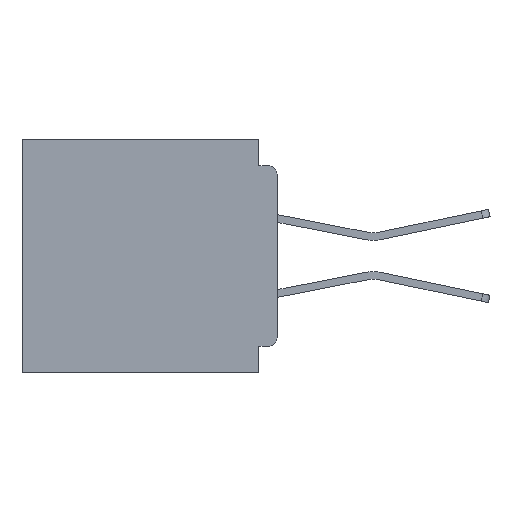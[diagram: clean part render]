
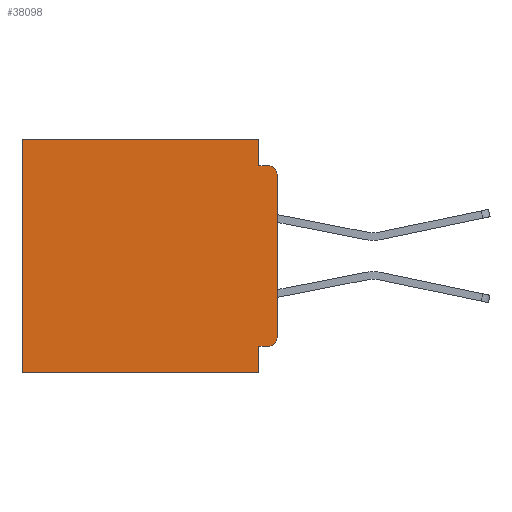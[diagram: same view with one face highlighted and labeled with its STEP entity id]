
A CAD part, left-side view. The second image highlights one B-rep face of the part: STEP entity #38098.
In plain terms, the highlighted planar face has unit normal (-1, 0, 0).
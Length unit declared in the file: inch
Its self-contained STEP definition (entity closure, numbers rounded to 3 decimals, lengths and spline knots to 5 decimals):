
#147 = FACE_OUTER_BOUND ( 'NONE', #43407, .T. ) ;
#606 = EDGE_CURVE ( 'NONE', #39332, #37207, #25156, .T. ) ;
#1272 = CARTESIAN_POINT ( 'NONE',  ( 0.3, 0.437, -0.4 ) ) ;
#1820 = EDGE_CURVE ( 'NONE', #10817, #36808, #22359, .T. ) ;
#2130 = DIRECTION ( 'NONE',  ( 0., 0., -1. ) ) ;
#2560 = ORIENTED_EDGE ( 'NONE', *, *, #606, .F. ) ;
#2570 = DIRECTION ( 'NONE',  ( 0., 0., -1. ) ) ;
#2652 = CIRCLE ( 'NONE', #17089, 0.015 ) ;
#2797 = DIRECTION ( 'NONE',  ( -1., 0., 0. ) ) ;
#3921 = ORIENTED_EDGE ( 'NONE', *, *, #14680, .F. ) ;
#4064 = ORIENTED_EDGE ( 'NONE', *, *, #9618, .T. ) ;
#5972 = DIRECTION ( 'NONE',  ( 0., 0., -1. ) ) ;
#6130 = VERTEX_POINT ( 'NONE', #18935 ) ;
#6526 = DIRECTION ( 'NONE',  ( 0., -1., 0. ) ) ;
#8549 = CARTESIAN_POINT ( 'NONE',  ( 0.3, 0., -0.4 ) ) ;
#8868 = VERTEX_POINT ( 'NONE', #12623 ) ;
#8914 = DIRECTION ( 'NONE',  ( 0., 0., -1. ) ) ;
#9393 = CARTESIAN_POINT ( 'NONE',  ( 0.3, 0.437, 0. ) ) ;
#9618 = EDGE_CURVE ( 'NONE', #10817, #8868, #2652, .T. ) ;
#10704 = VERTEX_POINT ( 'NONE', #26152 ) ;
#10817 = VERTEX_POINT ( 'NONE', #30225 ) ;
#11202 = VECTOR ( 'NONE', #26905, 39.37008 ) ;
#11681 = ORIENTED_EDGE ( 'NONE', *, *, #40359, .T. ) ;
#11682 = CARTESIAN_POINT ( 'NONE',  ( 0.3, 0.031, 0. ) ) ;
#12623 = CARTESIAN_POINT ( 'NONE',  ( 0.3, 0.015, -0.045 ) ) ;
#12744 = CARTESIAN_POINT ( 'NONE',  ( 0.3, 0., -0.4 ) ) ;
#12947 = CARTESIAN_POINT ( 'NONE',  ( 0.3, 0., 0. ) ) ;
#14680 = EDGE_CURVE ( 'NONE', #10704, #8868, #37393, .T. ) ;
#14986 = CARTESIAN_POINT ( 'NONE',  ( 0.3, 0.015, -0.34 ) ) ;
#15662 = EDGE_CURVE ( 'NONE', #21850, #10704, #32672, .T. ) ;
#16188 = CARTESIAN_POINT ( 'NONE',  ( 0.3, 0., -0.34 ) ) ;
#16303 = EDGE_CURVE ( 'NONE', #28092, #37207, #42016, .T. ) ;
#16659 = CARTESIAN_POINT ( 'NONE',  ( 0.3, 0.015, -0.355 ) ) ;
#17089 = AXIS2_PLACEMENT_3D ( 'NONE', #23402, #2797, #26845 ) ;
#17104 = VECTOR ( 'NONE', #6526, 39.37008 ) ;
#18450 = DIRECTION ( 'NONE',  ( 0., 0., -1. ) ) ;
#18935 = CARTESIAN_POINT ( 'NONE',  ( 0.3, 0.031, -0.355 ) ) ;
#19880 = VECTOR ( 'NONE', #36865, 39.37008 ) ;
#19909 = ORIENTED_EDGE ( 'NONE', *, *, #16303, .T. ) ;
#20310 = ORIENTED_EDGE ( 'NONE', *, *, #31011, .F. ) ;
#20761 = EDGE_CURVE ( 'NONE', #22041, #6130, #40576, .T. ) ;
#21850 = VERTEX_POINT ( 'NONE', #11682 ) ;
#22041 = VERTEX_POINT ( 'NONE', #16659 ) ;
#22345 = AXIS2_PLACEMENT_3D ( 'NONE', #14986, #38849, #18450 ) ;
#22359 = LINE ( 'NONE', #8549, #39309 ) ;
#22514 = VECTOR ( 'NONE', #8914, 39.37008 ) ;
#23038 = PLANE ( 'NONE',  #38952 ) ;
#23187 = DIRECTION ( 'NONE',  ( 1., 0., 0. ) ) ;
#23402 = CARTESIAN_POINT ( 'NONE',  ( 0.3, 0.015, -0.06 ) ) ;
#23464 = CARTESIAN_POINT ( 'NONE',  ( 0.3, 0., -0.355 ) ) ;
#24066 = CIRCLE ( 'NONE', #22345, 0.015 ) ;
#25050 = ORIENTED_EDGE ( 'NONE', *, *, #42413, .T. ) ;
#25156 = LINE ( 'NONE', #28033, #33139 ) ;
#25343 = VECTOR ( 'NONE', #31512, 39.37008 ) ;
#26152 = CARTESIAN_POINT ( 'NONE',  ( 0.3, 0.031, -0.045 ) ) ;
#26845 = DIRECTION ( 'NONE',  ( 0., 0., -1. ) ) ;
#26905 = DIRECTION ( 'NONE',  ( 0., 1., 0. ) ) ;
#28033 = CARTESIAN_POINT ( 'NONE',  ( 0.3, 0., -0.4 ) ) ;
#28092 = VERTEX_POINT ( 'NONE', #9393 ) ;
#29003 = LINE ( 'NONE', #12947, #19880 ) ;
#29504 = CARTESIAN_POINT ( 'NONE',  ( 0.3, 0.437, -0.4 ) ) ;
#29840 = ORIENTED_EDGE ( 'NONE', *, *, #1820, .F. ) ;
#30225 = CARTESIAN_POINT ( 'NONE',  ( 0.3, 0., -0.06 ) ) ;
#31011 = EDGE_CURVE ( 'NONE', #6130, #39332, #34375, .T. ) ;
#31512 = DIRECTION ( 'NONE',  ( 0., 0., -1. ) ) ;
#32672 = LINE ( 'NONE', #39532, #22514 ) ;
#33123 = VECTOR ( 'NONE', #2130, 39.37008 ) ;
#33139 = VECTOR ( 'NONE', #33577, 39.37008 ) ;
#33577 = DIRECTION ( 'NONE',  ( 0., 1., 0. ) ) ;
#34375 = LINE ( 'NONE', #34872, #25343 ) ;
#34872 = CARTESIAN_POINT ( 'NONE',  ( 0.3, 0.031, -0.4 ) ) ;
#34921 = CARTESIAN_POINT ( 'NONE',  ( 0.3, 0.031, -0.4 ) ) ;
#36400 = ORIENTED_EDGE ( 'NONE', *, *, #15662, .F. ) ;
#36808 = VERTEX_POINT ( 'NONE', #16188 ) ;
#36849 = ORIENTED_EDGE ( 'NONE', *, *, #20761, .F. ) ;
#36865 = DIRECTION ( 'NONE',  ( 0., 1., 0. ) ) ;
#37172 = CARTESIAN_POINT ( 'NONE',  ( 0.3, 0., -0.045 ) ) ;
#37207 = VERTEX_POINT ( 'NONE', #1272 ) ;
#37393 = LINE ( 'NONE', #37172, #17104 ) ;
#38098 = ADVANCED_FACE ( 'NONE', ( #147 ), #23038, .F. ) ;
#38849 = DIRECTION ( 'NONE',  ( -1., 0., 0. ) ) ;
#38952 = AXIS2_PLACEMENT_3D ( 'NONE', #12744, #23187, #2570 ) ;
#39309 = VECTOR ( 'NONE', #5972, 39.37008 ) ;
#39332 = VERTEX_POINT ( 'NONE', #34921 ) ;
#39532 = CARTESIAN_POINT ( 'NONE',  ( 0.3, 0.031, 0. ) ) ;
#40359 = EDGE_CURVE ( 'NONE', #21850, #28092, #29003, .T. ) ;
#40576 = LINE ( 'NONE', #23464, #11202 ) ;
#42016 = LINE ( 'NONE', #29504, #33123 ) ;
#42413 = EDGE_CURVE ( 'NONE', #22041, #36808, #24066, .T. ) ;
#43407 = EDGE_LOOP ( 'NONE', ( #29840, #4064, #3921, #36400, #11681, #19909, #2560, #20310, #36849, #25050 ) ) ;
